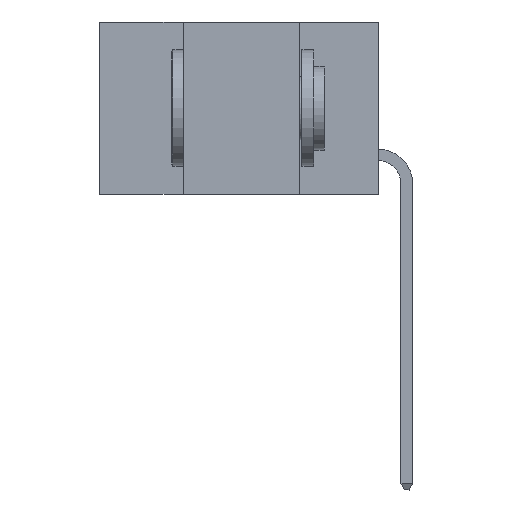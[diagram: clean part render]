
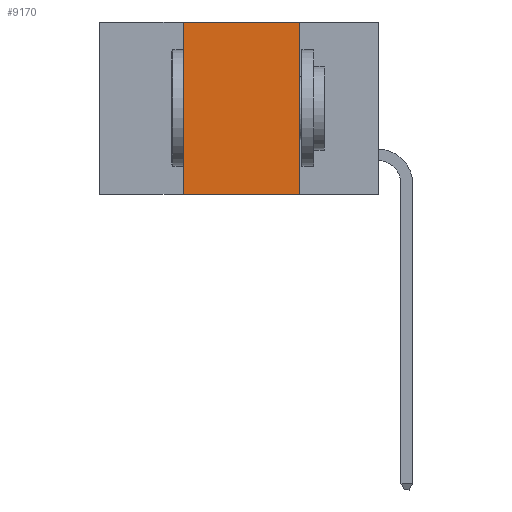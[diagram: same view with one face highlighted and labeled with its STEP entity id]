
A CAD part, left-side view. The second image highlights one B-rep face of the part: STEP entity #9170.
In plain terms, the highlighted planar face has unit normal (-1, 0, 0).
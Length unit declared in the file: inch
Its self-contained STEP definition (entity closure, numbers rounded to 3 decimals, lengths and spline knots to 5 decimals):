
#35 = EDGE_CURVE ( 'NONE', #744, #749, #4528, .T. ) ;
#77 = CARTESIAN_POINT ( 'NONE',  ( 0., 0.6, -0.37 ) ) ;
#645 = VECTOR ( 'NONE', #5195, 39.37008 ) ;
#744 = VERTEX_POINT ( 'NONE', #2601 ) ;
#749 = VERTEX_POINT ( 'NONE', #2738 ) ;
#934 = DIRECTION ( 'NONE',  ( 0., 0., -1. ) ) ;
#2091 = CARTESIAN_POINT ( 'NONE',  ( 0., 0.6, 0. ) ) ;
#2394 = VECTOR ( 'NONE', #6746, 39.37008 ) ;
#2601 = CARTESIAN_POINT ( 'NONE',  ( 0., 0.42, -0.37 ) ) ;
#2738 = CARTESIAN_POINT ( 'NONE',  ( 0., 0.42, 0. ) ) ;
#2882 = DIRECTION ( 'NONE',  ( 0., 0., -1. ) ) ;
#3041 = LINE ( 'NONE', #77, #9460 ) ;
#3326 = ORIENTED_EDGE ( 'NONE', *, *, #8657, .F. ) ;
#3332 = EDGE_CURVE ( 'NONE', #744, #8938, #3041, .T. ) ;
#3520 = VECTOR ( 'NONE', #934, 39.37008 ) ;
#4067 = ORIENTED_EDGE ( 'NONE', *, *, #3332, .T. ) ;
#4488 = LINE ( 'NONE', #7500, #2394 ) ;
#4528 = LINE ( 'NONE', #8334, #645 ) ;
#4764 = VERTEX_POINT ( 'NONE', #7513 ) ;
#4795 = EDGE_LOOP ( 'NONE', ( #9269, #3326, #7079, #4067 ) ) ;
#5195 = DIRECTION ( 'NONE',  ( 0., 0., 1. ) ) ;
#5516 = CARTESIAN_POINT ( 'NONE',  ( 0., 0.17, -0.37 ) ) ;
#5542 = FACE_OUTER_BOUND ( 'NONE', #4795, .T. ) ;
#5930 = PLANE ( 'NONE',  #9167 ) ;
#6232 = DIRECTION ( 'NONE',  ( 0., -1., 0. ) ) ;
#6746 = DIRECTION ( 'NONE',  ( 0., -1., 0. ) ) ;
#7079 = ORIENTED_EDGE ( 'NONE', *, *, #35, .F. ) ;
#7500 = CARTESIAN_POINT ( 'NONE',  ( 0., 0.6, 0. ) ) ;
#7513 = CARTESIAN_POINT ( 'NONE',  ( 0., 0.17, 0. ) ) ;
#7524 = DIRECTION ( 'NONE',  ( 1., 0., 0. ) ) ;
#8320 = EDGE_CURVE ( 'NONE', #4764, #8938, #9682, .T. ) ;
#8334 = CARTESIAN_POINT ( 'NONE',  ( 0., 0.42, 0. ) ) ;
#8657 = EDGE_CURVE ( 'NONE', #749, #4764, #4488, .T. ) ;
#8664 = CARTESIAN_POINT ( 'NONE',  ( 0., 0.17, 0. ) ) ;
#8938 = VERTEX_POINT ( 'NONE', #5516 ) ;
#9167 = AXIS2_PLACEMENT_3D ( 'NONE', #2091, #7524, #2882 ) ;
#9170 = ADVANCED_FACE ( 'NONE', ( #5542 ), #5930, .F. ) ;
#9269 = ORIENTED_EDGE ( 'NONE', *, *, #8320, .F. ) ;
#9460 = VECTOR ( 'NONE', #6232, 39.37008 ) ;
#9682 = LINE ( 'NONE', #8664, #3520 ) ;
